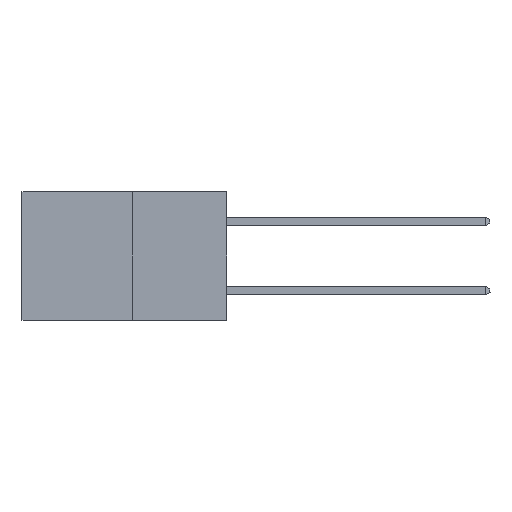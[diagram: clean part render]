
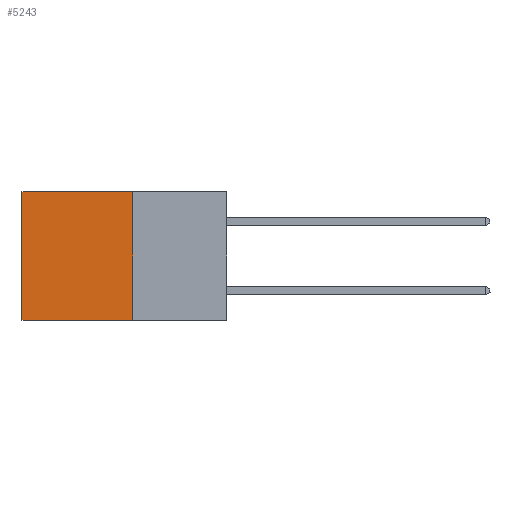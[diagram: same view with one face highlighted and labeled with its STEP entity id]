
A CAD part, left-side view. The second image highlights one B-rep face of the part: STEP entity #5243.
In plain terms, the highlighted planar face has unit normal (-1, 0, 0).
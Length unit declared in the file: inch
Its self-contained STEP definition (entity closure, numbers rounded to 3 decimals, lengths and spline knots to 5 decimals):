
#181 = ORIENTED_EDGE ( 'NONE', *, *, #4096, .T. ) ;
#188 = ORIENTED_EDGE ( 'NONE', *, *, #4761, .F. ) ;
#204 = ORIENTED_EDGE ( 'NONE', *, *, #896, .F. ) ;
#256 = ORIENTED_EDGE ( 'NONE', *, *, #5723, .T. ) ;
#430 = CARTESIAN_POINT ( 'NONE',  ( 0.277, 0.59, 0. ) ) ;
#799 = VECTOR ( 'NONE', #9245, 39.37008 ) ;
#896 = EDGE_CURVE ( 'NONE', #3012, #6105, #3650, .T. ) ;
#1696 = DIRECTION ( 'NONE',  ( 0., 1., 0. ) ) ;
#2172 = PLANE ( 'NONE',  #8930 ) ;
#2648 = VECTOR ( 'NONE', #6936, 39.37008 ) ;
#2821 = CARTESIAN_POINT ( 'NONE',  ( 0.277, 0.27, -0.37 ) ) ;
#3012 = VERTEX_POINT ( 'NONE', #9747 ) ;
#3120 = CARTESIAN_POINT ( 'NONE',  ( 0.277, 0.27, 0. ) ) ;
#3650 = LINE ( 'NONE', #2821, #5508 ) ;
#4096 = EDGE_CURVE ( 'NONE', #8786, #7958, #7208, .T. ) ;
#4761 = EDGE_CURVE ( 'NONE', #8786, #3012, #8202, .T. ) ;
#4777 = LINE ( 'NONE', #9092, #2648 ) ;
#5053 = DIRECTION ( 'NONE',  ( 1., 0., 0. ) ) ;
#5243 = ADVANCED_FACE ( 'NONE', ( #8287 ), #2172, .F. ) ;
#5508 = VECTOR ( 'NONE', #1696, 39.37008 ) ;
#5723 = EDGE_CURVE ( 'NONE', #7958, #6105, #4777, .T. ) ;
#5859 = EDGE_LOOP ( 'NONE', ( #256, #204, #188, #181 ) ) ;
#6105 = VERTEX_POINT ( 'NONE', #9281 ) ;
#6835 = CARTESIAN_POINT ( 'NONE',  ( 0.277, 0.27, -0.37 ) ) ;
#6936 = DIRECTION ( 'NONE',  ( 0., 0., -1. ) ) ;
#7208 = LINE ( 'NONE', #9216, #799 ) ;
#7958 = VERTEX_POINT ( 'NONE', #430 ) ;
#8202 = LINE ( 'NONE', #9386, #10010 ) ;
#8287 = FACE_OUTER_BOUND ( 'NONE', #5859, .T. ) ;
#8525 = DIRECTION ( 'NONE',  ( 0., 0., -1. ) ) ;
#8786 = VERTEX_POINT ( 'NONE', #3120 ) ;
#8930 = AXIS2_PLACEMENT_3D ( 'NONE', #6835, #5053, #8525 ) ;
#9092 = CARTESIAN_POINT ( 'NONE',  ( 0.277, 0.59, -0.37 ) ) ;
#9216 = CARTESIAN_POINT ( 'NONE',  ( 0.277, 0.27, 0. ) ) ;
#9245 = DIRECTION ( 'NONE',  ( 0., 1., 0. ) ) ;
#9281 = CARTESIAN_POINT ( 'NONE',  ( 0.277, 0.59, -0.37 ) ) ;
#9386 = CARTESIAN_POINT ( 'NONE',  ( 0.277, 0.27, -0.37 ) ) ;
#9560 = DIRECTION ( 'NONE',  ( 0., 0., -1. ) ) ;
#9747 = CARTESIAN_POINT ( 'NONE',  ( 0.277, 0.27, -0.37 ) ) ;
#10010 = VECTOR ( 'NONE', #9560, 39.37008 ) ;
